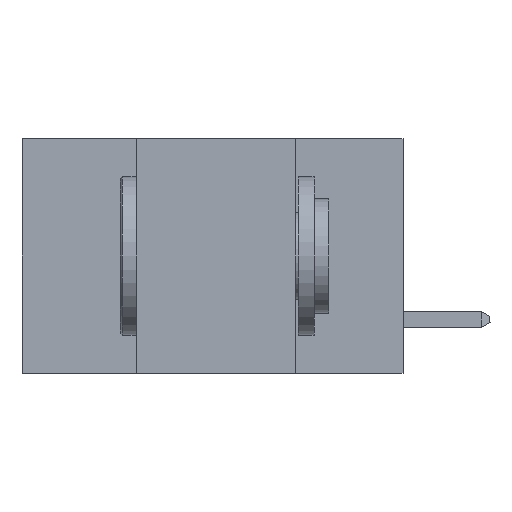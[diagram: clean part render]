
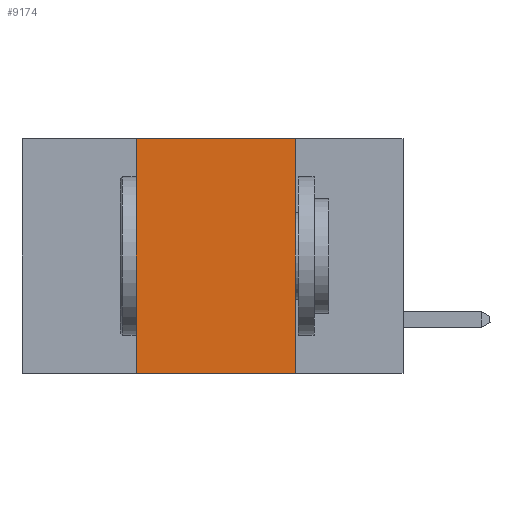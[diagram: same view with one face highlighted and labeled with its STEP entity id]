
A CAD part, left-side view. The second image highlights one B-rep face of the part: STEP entity #9174.
In plain terms, the highlighted planar face has unit normal (-1, 0, 0).
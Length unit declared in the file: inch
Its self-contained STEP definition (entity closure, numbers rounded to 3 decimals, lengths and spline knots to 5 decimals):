
#412 = EDGE_CURVE ( 'NONE', #4660, #25075, #877, .T. ) ;
#877 = LINE ( 'NONE', #1867, #29376 ) ;
#1834 = DIRECTION ( 'NONE',  ( 0., -1., 0. ) ) ;
#1867 = CARTESIAN_POINT ( 'NONE',  ( 0., 0.6, 0. ) ) ;
#3597 = CARTESIAN_POINT ( 'NONE',  ( 0., 0.6, 0. ) ) ;
#4660 = VERTEX_POINT ( 'NONE', #19920 ) ;
#5673 = VERTEX_POINT ( 'NONE', #29234 ) ;
#6726 = DIRECTION ( 'NONE',  ( 0., 0., -1. ) ) ;
#8650 = ORIENTED_EDGE ( 'NONE', *, *, #24422, .T. ) ;
#8811 = ORIENTED_EDGE ( 'NONE', *, *, #29686, .F. ) ;
#9174 = ADVANCED_FACE ( 'NONE', ( #31132 ), #15853, .F. ) ;
#10205 = VECTOR ( 'NONE', #36945, 39.37008 ) ;
#11203 = CARTESIAN_POINT ( 'NONE',  ( 0., 0.42, -0.37 ) ) ;
#13132 = CARTESIAN_POINT ( 'NONE',  ( 0., 0.17, 0. ) ) ;
#15586 = CARTESIAN_POINT ( 'NONE',  ( 0., 0.6, -0.37 ) ) ;
#15799 = ORIENTED_EDGE ( 'NONE', *, *, #37712, .F. ) ;
#15853 = PLANE ( 'NONE',  #38608 ) ;
#17777 = VECTOR ( 'NONE', #18600, 39.37008 ) ;
#18600 = DIRECTION ( 'NONE',  ( 0., -1., 0. ) ) ;
#19124 = ORIENTED_EDGE ( 'NONE', *, *, #412, .F. ) ;
#19861 = VERTEX_POINT ( 'NONE', #11203 ) ;
#19920 = CARTESIAN_POINT ( 'NONE',  ( 0., 0.42, 0. ) ) ;
#22028 = CARTESIAN_POINT ( 'NONE',  ( 0., 0.17, 0. ) ) ;
#24094 = LINE ( 'NONE', #32787, #39030 ) ;
#24422 = EDGE_CURVE ( 'NONE', #19861, #5673, #32777, .T. ) ;
#24817 = EDGE_LOOP ( 'NONE', ( #15799, #19124, #8811, #8650 ) ) ;
#24907 = DIRECTION ( 'NONE',  ( 1., 0., 0. ) ) ;
#25075 = VERTEX_POINT ( 'NONE', #13132 ) ;
#25302 = LINE ( 'NONE', #22028, #10205 ) ;
#29234 = CARTESIAN_POINT ( 'NONE',  ( 0., 0.17, -0.37 ) ) ;
#29376 = VECTOR ( 'NONE', #1834, 39.37008 ) ;
#29686 = EDGE_CURVE ( 'NONE', #19861, #4660, #24094, .T. ) ;
#29771 = DIRECTION ( 'NONE',  ( 0., 0., 1. ) ) ;
#31132 = FACE_OUTER_BOUND ( 'NONE', #24817, .T. ) ;
#32777 = LINE ( 'NONE', #15586, #17777 ) ;
#32787 = CARTESIAN_POINT ( 'NONE',  ( 0., 0.42, 0. ) ) ;
#36945 = DIRECTION ( 'NONE',  ( 0., 0., -1. ) ) ;
#37712 = EDGE_CURVE ( 'NONE', #25075, #5673, #25302, .T. ) ;
#38608 = AXIS2_PLACEMENT_3D ( 'NONE', #3597, #24907, #6726 ) ;
#39030 = VECTOR ( 'NONE', #29771, 39.37008 ) ;
